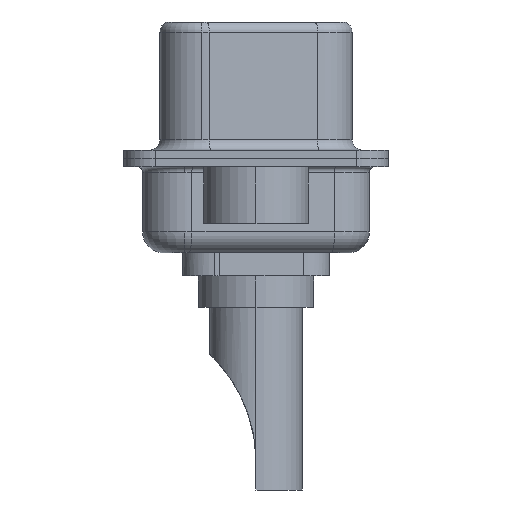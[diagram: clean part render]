
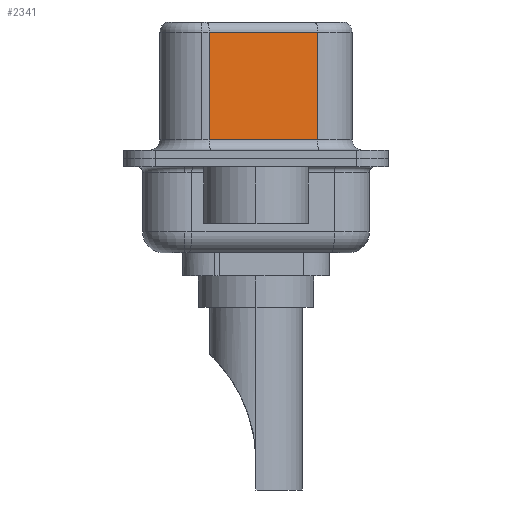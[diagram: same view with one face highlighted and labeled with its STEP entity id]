
A CAD part, left-side view. The second image highlights one B-rep face of the part: STEP entity #2341.
In plain terms, the highlighted planar face has unit normal (-0.985, -0.174, 0).
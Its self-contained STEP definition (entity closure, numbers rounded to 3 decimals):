
#2173 = EDGE_CURVE ( 'NONE', #14444, #14766, #14068, .T. ) ;
#2341 = ADVANCED_FACE ( 'NONE', ( #15147 ), #10011, .F. ) ;
#2884 = LINE ( 'NONE', #13132, #6769 ) ;
#3046 = DIRECTION ( 'NONE',  ( 0.174, -0.985, 0. ) ) ;
#3642 = EDGE_LOOP ( 'NONE', ( #16204, #5260, #10570, #9596 ) ) ;
#4051 = CARTESIAN_POINT ( 'NONE',  ( 4.585, -2.927, 6.52 ) ) ;
#5260 = ORIENTED_EDGE ( 'NONE', *, *, #2173, .T. ) ;
#5461 = CARTESIAN_POINT ( 'NONE',  ( 4.585, -2.927, 6.52 ) ) ;
#6769 = VECTOR ( 'NONE', #3046, 1000. ) ;
#7201 = LINE ( 'NONE', #5461, #18135 ) ;
#7396 = EDGE_CURVE ( 'NONE', #13448, #8379, #2884, .T. ) ;
#8366 = EDGE_CURVE ( 'NONE', #14444, #8379, #7201, .T. ) ;
#8379 = VERTEX_POINT ( 'NONE', #14094 ) ;
#8957 = VECTOR ( 'NONE', #14896, 1000. ) ;
#9160 = DIRECTION ( 'NONE',  ( -0.174, 0.985, 0. ) ) ;
#9183 = CARTESIAN_POINT ( 'NONE',  ( 3.675, 2.233, 6.52 ) ) ;
#9596 = ORIENTED_EDGE ( 'NONE', *, *, #7396, .T. ) ;
#9707 = DIRECTION ( 'NONE',  ( 0.985, 0.174, 0. ) ) ;
#9840 = DIRECTION ( 'NONE',  ( -0.174, 0.985, 0. ) ) ;
#10011 = PLANE ( 'NONE',  #10092 ) ;
#10092 = AXIS2_PLACEMENT_3D ( 'NONE', #4051, #9707, #9840 ) ;
#10570 = ORIENTED_EDGE ( 'NONE', *, *, #18094, .T. ) ;
#11133 = VECTOR ( 'NONE', #9160, 1000. ) ;
#12368 = CARTESIAN_POINT ( 'NONE',  ( 3.675, 2.233, 6.02 ) ) ;
#13132 = CARTESIAN_POINT ( 'NONE',  ( 4.585, -2.927, 0.9 ) ) ;
#13448 = VERTEX_POINT ( 'NONE', #16222 ) ;
#14068 = LINE ( 'NONE', #16235, #11133 ) ;
#14094 = CARTESIAN_POINT ( 'NONE',  ( 4.585, -2.927, 0.9 ) ) ;
#14444 = VERTEX_POINT ( 'NONE', #15837 ) ;
#14766 = VERTEX_POINT ( 'NONE', #12368 ) ;
#14896 = DIRECTION ( 'NONE',  ( 0., 0., -1. ) ) ;
#15147 = FACE_OUTER_BOUND ( 'NONE', #3642, .T. ) ;
#15437 = DIRECTION ( 'NONE',  ( 0., 0., -1. ) ) ;
#15837 = CARTESIAN_POINT ( 'NONE',  ( 4.585, -2.927, 6.02 ) ) ;
#16204 = ORIENTED_EDGE ( 'NONE', *, *, #8366, .F. ) ;
#16222 = CARTESIAN_POINT ( 'NONE',  ( 3.675, 2.233, 0.9 ) ) ;
#16235 = CARTESIAN_POINT ( 'NONE',  ( 4.585, -2.927, 6.02 ) ) ;
#17420 = LINE ( 'NONE', #9183, #8957 ) ;
#18094 = EDGE_CURVE ( 'NONE', #14766, #13448, #17420, .T. ) ;
#18135 = VECTOR ( 'NONE', #15437, 1000. ) ;
